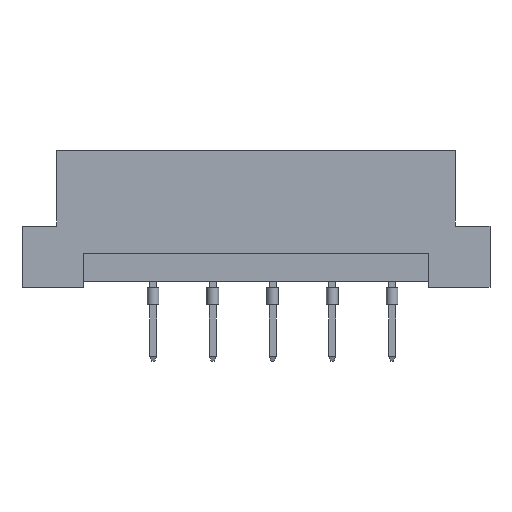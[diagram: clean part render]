
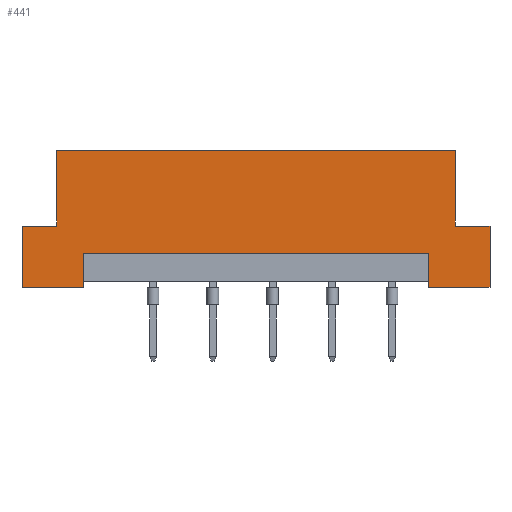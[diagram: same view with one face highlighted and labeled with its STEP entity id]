
A CAD part, front view. The second image highlights one B-rep face of the part: STEP entity #441.
In plain terms, the highlighted planar face has unit normal (0, -1, 0).
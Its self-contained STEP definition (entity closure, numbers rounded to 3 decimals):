
#61 = VERTEX_POINT ( 'NONE', #339 ) ;
#133 = LINE ( 'NONE', #2304, #6615 ) ;
#194 = VERTEX_POINT ( 'NONE', #544 ) ;
#267 = ORIENTED_EDGE ( 'NONE', *, *, #5327, .F. ) ;
#312 = DIRECTION ( 'NONE',  ( 1., 0., 0. ) ) ;
#322 = VECTOR ( 'NONE', #3782, 1000. ) ;
#339 = CARTESIAN_POINT ( 'NONE',  ( 16.94, 0., 11.6 ) ) ;
#441 = ADVANCED_FACE ( 'NONE', ( #2540 ), #1472, .F. ) ;
#442 = VECTOR ( 'NONE', #4958, 1000. ) ;
#479 = AXIS2_PLACEMENT_3D ( 'NONE', #4797, #6336, #4732 ) ;
#486 = VECTOR ( 'NONE', #2982, 1000. ) ;
#544 = CARTESIAN_POINT ( 'NONE',  ( 19.9, 0., 5.2 ) ) ;
#576 = CARTESIAN_POINT ( 'NONE',  ( -14.69, 0., 2.9 ) ) ;
#596 = CARTESIAN_POINT ( 'NONE',  ( -14.69, 0., 0.5 ) ) ;
#632 = LINE ( 'NONE', #2771, #6590 ) ;
#638 = ORIENTED_EDGE ( 'NONE', *, *, #6580, .T. ) ;
#796 = VERTEX_POINT ( 'NONE', #5079 ) ;
#801 = CARTESIAN_POINT ( 'NONE',  ( -19.9, 0., 5.2 ) ) ;
#1067 = LINE ( 'NONE', #2671, #1798 ) ;
#1079 = CARTESIAN_POINT ( 'NONE',  ( -19.9, 0., 0. ) ) ;
#1221 = LINE ( 'NONE', #1079, #3421 ) ;
#1449 = EDGE_CURVE ( 'NONE', #3500, #796, #1221, .T. ) ;
#1472 = PLANE ( 'NONE',  #479 ) ;
#1628 = CARTESIAN_POINT ( 'NONE',  ( -19.9, 0., 0. ) ) ;
#1655 = EDGE_CURVE ( 'NONE', #796, #2775, #3555, .T. ) ;
#1798 = VECTOR ( 'NONE', #2176, 1000. ) ;
#1821 = CARTESIAN_POINT ( 'NONE',  ( 14.69, 0., 2.9 ) ) ;
#1853 = LINE ( 'NONE', #5039, #6487 ) ;
#1871 = VERTEX_POINT ( 'NONE', #576 ) ;
#2091 = CARTESIAN_POINT ( 'NONE',  ( 19.9, 0., 0. ) ) ;
#2156 = ORIENTED_EDGE ( 'NONE', *, *, #2611, .F. ) ;
#2176 = DIRECTION ( 'NONE',  ( -1., 0., 0. ) ) ;
#2231 = CARTESIAN_POINT ( 'NONE',  ( -16.94, 0., 5.2 ) ) ;
#2263 = EDGE_CURVE ( 'NONE', #194, #6261, #3581, .T. ) ;
#2287 = EDGE_LOOP ( 'NONE', ( #6445, #638, #267, #5353, #3454, #5427, #2156, #3466, #4409, #6093, #3018, #5963 ) ) ;
#2304 = CARTESIAN_POINT ( 'NONE',  ( 14.69, 0., 2.9 ) ) ;
#2378 = CARTESIAN_POINT ( 'NONE',  ( -14.69, 0., 0. ) ) ;
#2479 = DIRECTION ( 'NONE',  ( 0., 0., -1. ) ) ;
#2493 = LINE ( 'NONE', #5250, #5790 ) ;
#2539 = DIRECTION ( 'NONE',  ( 1., 0., 0. ) ) ;
#2540 = FACE_OUTER_BOUND ( 'NONE', #2287, .T. ) ;
#2611 = EDGE_CURVE ( 'NONE', #3021, #61, #2493, .T. ) ;
#2671 = CARTESIAN_POINT ( 'NONE',  ( -19.9, 0., 0. ) ) ;
#2771 = CARTESIAN_POINT ( 'NONE',  ( 16.94, 0., 5.2 ) ) ;
#2775 = VERTEX_POINT ( 'NONE', #2231 ) ;
#2908 = EDGE_CURVE ( 'NONE', #4033, #1871, #133, .T. ) ;
#2910 = CARTESIAN_POINT ( 'NONE',  ( 14.69, 0., 0.5 ) ) ;
#2914 = VERTEX_POINT ( 'NONE', #6640 ) ;
#2982 = DIRECTION ( 'NONE',  ( 1., 0., 0. ) ) ;
#3018 = ORIENTED_EDGE ( 'NONE', *, *, #5852, .F. ) ;
#3021 = VERTEX_POINT ( 'NONE', #6889 ) ;
#3037 = VERTEX_POINT ( 'NONE', #2378 ) ;
#3108 = CARTESIAN_POINT ( 'NONE',  ( 19.9, 0., 5.2 ) ) ;
#3421 = VECTOR ( 'NONE', #5054, 1000. ) ;
#3454 = ORIENTED_EDGE ( 'NONE', *, *, #5161, .F. ) ;
#3466 = ORIENTED_EDGE ( 'NONE', *, *, #3794, .F. ) ;
#3500 = VERTEX_POINT ( 'NONE', #3583 ) ;
#3555 = LINE ( 'NONE', #801, #486 ) ;
#3559 = LINE ( 'NONE', #2910, #5798 ) ;
#3581 = LINE ( 'NONE', #6325, #5995 ) ;
#3583 = CARTESIAN_POINT ( 'NONE',  ( -19.9, 0., 0. ) ) ;
#3782 = DIRECTION ( 'NONE',  ( -1., 0., 0. ) ) ;
#3794 = EDGE_CURVE ( 'NONE', #2775, #3021, #1853, .T. ) ;
#3816 = LINE ( 'NONE', #1628, #322 ) ;
#4033 = VERTEX_POINT ( 'NONE', #1821 ) ;
#4389 = DIRECTION ( 'NONE',  ( 0., 0., 1. ) ) ;
#4409 = ORIENTED_EDGE ( 'NONE', *, *, #1655, .F. ) ;
#4488 = EDGE_CURVE ( 'NONE', #4587, #61, #632, .T. ) ;
#4495 = DIRECTION ( 'NONE',  ( -1., 0., 0. ) ) ;
#4538 = DIRECTION ( 'NONE',  ( 0., 0., 1. ) ) ;
#4587 = VERTEX_POINT ( 'NONE', #6681 ) ;
#4732 = DIRECTION ( 'NONE',  ( 0., 0., 1. ) ) ;
#4762 = LINE ( 'NONE', #3108, #6476 ) ;
#4797 = CARTESIAN_POINT ( 'NONE',  ( -19.9, 0., 11.6 ) ) ;
#4819 = DIRECTION ( 'NONE',  ( 0., 0., -1. ) ) ;
#4958 = DIRECTION ( 'NONE',  ( 0., 0., -1. ) ) ;
#5039 = CARTESIAN_POINT ( 'NONE',  ( -16.94, 0., 5.2 ) ) ;
#5054 = DIRECTION ( 'NONE',  ( 0., 0., 1. ) ) ;
#5079 = CARTESIAN_POINT ( 'NONE',  ( -19.9, 0., 5.2 ) ) ;
#5161 = EDGE_CURVE ( 'NONE', #4587, #194, #4762, .T. ) ;
#5250 = CARTESIAN_POINT ( 'NONE',  ( -19.9, 0., 11.6 ) ) ;
#5327 = EDGE_CURVE ( 'NONE', #6261, #2914, #1067, .T. ) ;
#5353 = ORIENTED_EDGE ( 'NONE', *, *, #2263, .F. ) ;
#5427 = ORIENTED_EDGE ( 'NONE', *, *, #4488, .T. ) ;
#5790 = VECTOR ( 'NONE', #312, 1000. ) ;
#5798 = VECTOR ( 'NONE', #2479, 1000. ) ;
#5852 = EDGE_CURVE ( 'NONE', #3037, #3500, #3816, .T. ) ;
#5963 = ORIENTED_EDGE ( 'NONE', *, *, #5973, .F. ) ;
#5973 = EDGE_CURVE ( 'NONE', #1871, #3037, #6683, .T. ) ;
#5995 = VECTOR ( 'NONE', #4819, 1000. ) ;
#6093 = ORIENTED_EDGE ( 'NONE', *, *, #1449, .F. ) ;
#6261 = VERTEX_POINT ( 'NONE', #2091 ) ;
#6325 = CARTESIAN_POINT ( 'NONE',  ( 19.9, 0., 0. ) ) ;
#6336 = DIRECTION ( 'NONE',  ( 0., 1., 0. ) ) ;
#6445 = ORIENTED_EDGE ( 'NONE', *, *, #2908, .F. ) ;
#6476 = VECTOR ( 'NONE', #2539, 1000. ) ;
#6487 = VECTOR ( 'NONE', #4538, 1000. ) ;
#6580 = EDGE_CURVE ( 'NONE', #4033, #2914, #3559, .T. ) ;
#6590 = VECTOR ( 'NONE', #4389, 1000. ) ;
#6615 = VECTOR ( 'NONE', #4495, 1000. ) ;
#6640 = CARTESIAN_POINT ( 'NONE',  ( 14.69, 0., 0. ) ) ;
#6681 = CARTESIAN_POINT ( 'NONE',  ( 16.94, 0., 5.2 ) ) ;
#6683 = LINE ( 'NONE', #596, #442 ) ;
#6889 = CARTESIAN_POINT ( 'NONE',  ( -16.94, 0., 11.6 ) ) ;
